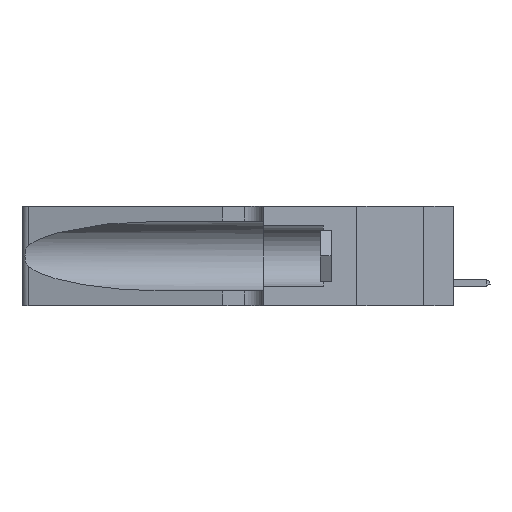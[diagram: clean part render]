
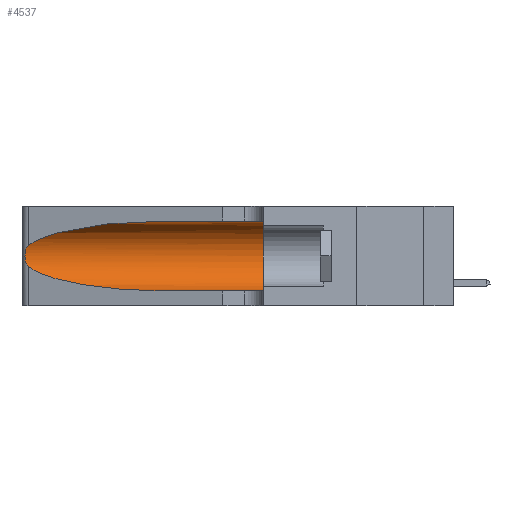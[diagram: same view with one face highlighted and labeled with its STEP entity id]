
A CAD part, left-side view. The second image highlights one B-rep face of the part: STEP entity #4537.
In plain terms, the highlighted cylindrical face has radius 3.308 mm (diameter 6.617 mm), a partial arc.
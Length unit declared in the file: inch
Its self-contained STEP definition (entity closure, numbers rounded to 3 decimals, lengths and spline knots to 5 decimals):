
#149 = ORIENTED_EDGE ( 'NONE', *, *, #193, .T. ) ;
#193 = EDGE_CURVE ( 'NONE', #44375, #28868, #29944, .T. ) ;
#1521 = CARTESIAN_POINT ( 'NONE',  ( 0.1305, 0.72297, 0.31525 ) ) ;
#2216 = CARTESIAN_POINT ( 'NONE',  ( 0.1305, 0.72297, 0.31525 ) ) ;
#2952 = CARTESIAN_POINT ( 'NONE',  ( 0.25787, 1.23484, 0.2124 ) ) ;
#3118 = CARTESIAN_POINT ( 'NONE',  ( 0.25487, 1.22718, 0.14631 ) ) ;
#3279 = CARTESIAN_POINT ( 'NONE',  ( 0.25639, 1.23184, 0.21858 ) ) ;
#4318 =( BOUNDED_CURVE ( )  B_SPLINE_CURVE ( 3, ( #1521, #27249, #5239, #35132 ),
 .UNSPECIFIED., .F., .F. ) 
 B_SPLINE_CURVE_WITH_KNOTS ( ( 4, 4 ),
 ( 1.5708, 2.84003 ),
 .UNSPECIFIED. ) 
 CURVE ( )  GEOMETRIC_REPRESENTATION_ITEM ( )  RATIONAL_B_SPLINE_CURVE ( ( 1., 0.87, 0.87, 1. ) ) 
 REPRESENTATION_ITEM ( '' )  );
#4537 = ADVANCED_FACE ( 'NONE', ( #39549 ), #28676, .F. ) ;
#5187 = CARTESIAN_POINT ( 'NONE',  ( 0.1305, 0.72297, 0.05475 ) ) ;
#5239 = CARTESIAN_POINT ( 'NONE',  ( 0.2373, 1.15595, 0.28018 ) ) ;
#5805 = LINE ( 'NONE', #42278, #31080 ) ;
#6030 = VERTEX_POINT ( 'NONE', #2216 ) ;
#6196 = CARTESIAN_POINT ( 'NONE',  ( 0.1305, 0.35, 0.31525 ) ) ;
#9522 = CARTESIAN_POINT ( 'NONE',  ( 0.1305, 0.35, 0.185 ) ) ;
#9714 = DIRECTION ( 'NONE',  ( 0., -1., 0. ) ) ;
#12168 = AXIS2_PLACEMENT_3D ( 'NONE', #9522, #25170, #13096 ) ;
#12190 = EDGE_LOOP ( 'NONE', ( #26220, #42479, #149, #12647, #13093, #25690 ) ) ;
#12647 = ORIENTED_EDGE ( 'NONE', *, *, #18971, .T. ) ;
#12888 = B_SPLINE_CURVE_WITH_KNOTS ( 'NONE', 3,
 ( #32156, #36514, #3279, #2952, #17763, #21440, #21605, #17925, #47060, #40204, #25148, #21765, #43720, #3118 ),
 .UNSPECIFIED., .F., .F.,
 ( 4, 2, 2, 2, 2, 2, 4 ),
 ( 0., 0.00027, 0.00053, 0.00107, 0.0016, 0.00187, 0.00214 ),
 .UNSPECIFIED. ) ;
#13093 = ORIENTED_EDGE ( 'NONE', *, *, #26048, .F. ) ;
#13096 = DIRECTION ( 'NONE',  ( 0., 0., 1. ) ) ;
#14716 = EDGE_CURVE ( 'NONE', #6030, #21798, #5805, .T. ) ;
#15042 = CARTESIAN_POINT ( 'NONE',  ( 0.25487, 1.22718, 0.14631 ) ) ;
#17312 = EDGE_CURVE ( 'NONE', #37646, #44375, #12888, .T. ) ;
#17763 = CARTESIAN_POINT ( 'NONE',  ( 0.25854, 1.2359, 0.20912 ) ) ;
#17925 = CARTESIAN_POINT ( 'NONE',  ( 0.26075, 1.23896, 0.178 ) ) ;
#18428 = DIRECTION ( 'NONE',  ( 0., -1., 0. ) ) ;
#18971 = EDGE_CURVE ( 'NONE', #28868, #32570, #35281, .T. ) ;
#21440 = CARTESIAN_POINT ( 'NONE',  ( 0.26018, 1.23835, 0.19895 ) ) ;
#21503 = DIRECTION ( 'NONE',  ( 0., -1., 0. ) ) ;
#21605 = CARTESIAN_POINT ( 'NONE',  ( 0.26075, 1.23896, 0.19203 ) ) ;
#21765 = CARTESIAN_POINT ( 'NONE',  ( 0.25639, 1.23186, 0.15144 ) ) ;
#21798 = VERTEX_POINT ( 'NONE', #6196 ) ;
#21943 = AXIS2_PLACEMENT_3D ( 'NONE', #32995, #18428, #40666 ) ;
#25148 = CARTESIAN_POINT ( 'NONE',  ( 0.25789, 1.23486, 0.15765 ) ) ;
#25170 = DIRECTION ( 'NONE',  ( 0., 1., 0. ) ) ;
#25690 = ORIENTED_EDGE ( 'NONE', *, *, #14716, .F. ) ;
#26048 = EDGE_CURVE ( 'NONE', #21798, #32570, #31472, .T. ) ;
#26220 = ORIENTED_EDGE ( 'NONE', *, *, #29262, .T. ) ;
#27249 = CARTESIAN_POINT ( 'NONE',  ( 0.18966, 0.96281, 0.31525 ) ) ;
#28676 = CYLINDRICAL_SURFACE ( 'NONE', #21943, 0.13025 ) ;
#28868 = VERTEX_POINT ( 'NONE', #5187 ) ;
#29262 = EDGE_CURVE ( 'NONE', #6030, #37646, #4318, .T. ) ;
#29944 =( BOUNDED_CURVE ( )  B_SPLINE_CURVE ( 3, ( #45775, #35082, #34747, #38412 ),
 .UNSPECIFIED., .F., .F. ) 
 B_SPLINE_CURVE_WITH_KNOTS ( ( 4, 4 ),
 ( 3.44316, 4.71239 ),
 .UNSPECIFIED. ) 
 CURVE ( )  GEOMETRIC_REPRESENTATION_ITEM ( )  RATIONAL_B_SPLINE_CURVE ( ( 1., 0.87, 0.87, 1. ) ) 
 REPRESENTATION_ITEM ( '' )  );
#30397 = CARTESIAN_POINT ( 'NONE',  ( 0.1305, 0.35, 0.05475 ) ) ;
#31080 = VECTOR ( 'NONE', #9714, 39.37008 ) ;
#31472 = CIRCLE ( 'NONE', #12168, 0.13025 ) ;
#32156 = CARTESIAN_POINT ( 'NONE',  ( 0.25487, 1.22718, 0.22369 ) ) ;
#32570 = VERTEX_POINT ( 'NONE', #30397 ) ;
#32995 = CARTESIAN_POINT ( 'NONE',  ( 0.1305, 1.61858, 0.185 ) ) ;
#34111 = CARTESIAN_POINT ( 'NONE',  ( 0.25487, 1.22718, 0.22369 ) ) ;
#34747 = CARTESIAN_POINT ( 'NONE',  ( 0.18966, 0.96281, 0.05475 ) ) ;
#35082 = CARTESIAN_POINT ( 'NONE',  ( 0.2373, 1.15595, 0.08982 ) ) ;
#35132 = CARTESIAN_POINT ( 'NONE',  ( 0.25487, 1.22718, 0.22369 ) ) ;
#35281 = LINE ( 'NONE', #39784, #42099 ) ;
#36514 = CARTESIAN_POINT ( 'NONE',  ( 0.25555, 1.22994, 0.2215 ) ) ;
#37646 = VERTEX_POINT ( 'NONE', #34111 ) ;
#38412 = CARTESIAN_POINT ( 'NONE',  ( 0.1305, 0.72297, 0.05475 ) ) ;
#39549 = FACE_OUTER_BOUND ( 'NONE', #12190, .T. ) ;
#39784 = CARTESIAN_POINT ( 'NONE',  ( 0.1305, 1.61858, 0.05475 ) ) ;
#40204 = CARTESIAN_POINT ( 'NONE',  ( 0.25856, 1.23593, 0.16098 ) ) ;
#40666 = DIRECTION ( 'NONE',  ( 0., 0., -1. ) ) ;
#42099 = VECTOR ( 'NONE', #21503, 39.37008 ) ;
#42278 = CARTESIAN_POINT ( 'NONE',  ( 0.1305, 1.61858, 0.31525 ) ) ;
#42479 = ORIENTED_EDGE ( 'NONE', *, *, #17312, .T. ) ;
#43720 = CARTESIAN_POINT ( 'NONE',  ( 0.25555, 1.22993, 0.14849 ) ) ;
#44375 = VERTEX_POINT ( 'NONE', #15042 ) ;
#45775 = CARTESIAN_POINT ( 'NONE',  ( 0.25487, 1.22718, 0.14631 ) ) ;
#47060 = CARTESIAN_POINT ( 'NONE',  ( 0.26017, 1.23833, 0.17102 ) ) ;
